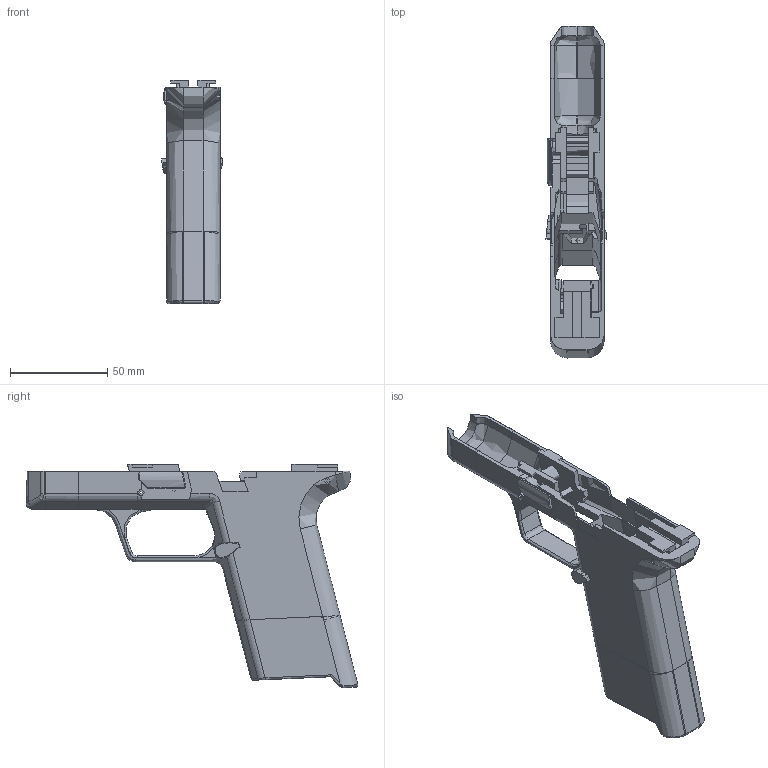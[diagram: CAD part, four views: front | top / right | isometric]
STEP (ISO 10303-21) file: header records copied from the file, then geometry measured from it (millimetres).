
FILE_DESCRIPTION(/* description */ (''),/* implementation_level */ '2;1');
FILE_NAME(/* name */ 'M&P 9 Assembly.step',/* time_stamp */ '2021-11-02T07:28:00-04:00',/* author */ (''),/* organization */ (''),/* preprocessor_version */ 'ST-DEVELOPER v18.1',/* originating_system */ 'Autodesk Translation Framework v10.10.0.1391',/* authorisation */ '');
FILE_SCHEMA (('AUTOMOTIVE_DESIGN { 1 0 10303 214 3 1 1 }'));
Length unit declared in the file: millimetre
Products named in the file (13): M&P 9 Reference; Rear Fire Control Group Pin; Front Locking Block Group Pin; Trigger Pin; Locking Block; Disassembly Lug; Rear Fire Control Group; Frame; Trigger Guard and Magwell; Fitment Section; Nose; Magazine Release Button; Full-Size Magwell Body
Assembly tree (12 placements, depth 4):
  M&P 9 Reference
    Rear Fire Control Group Pin
    Front Locking Block Group Pin
    Trigger Pin
    Locking Block
    Disassembly Lug
    Rear Fire Control Group
    Frame
      Trigger Guard and Magwell
      Fitment Section
        Nose
      Magazine Release Button
      Full-Size Magwell Body
Bounding box: 30.85 x 170.13 x 114.63 mm (x, y, z)
Volume: 102365.3 mm3; surface area: 57558.7 mm2
Topology: 12 solids, 12 shells, 608 faces, 1657 edges, 1059 vertices
Faces by surface type: plane 326, cylinder 185, bspline 75, torus 17, sphere 4, cone 1
Full cylindrical faces by diameter (mm): 1.35 x2, 2 x3, 3.15 x2, 3.18 x3, 3.2 x2, 3.361 x2, 3.5 x1, 3.55 x4, 4.7 x1, 6.3 x1, 7.7 x1, 8.8 x1, 9 x2
Entity records: 22075 total; most frequent: CARTESIAN_POINT 6358, ORIENTED_EDGE 3306, DIRECTION 3113, EDGE_CURVE 1653, VERTEX_POINT 1059, LINE 1049, VECTOR 1049, AXIS2_PLACEMENT_3D 1032
